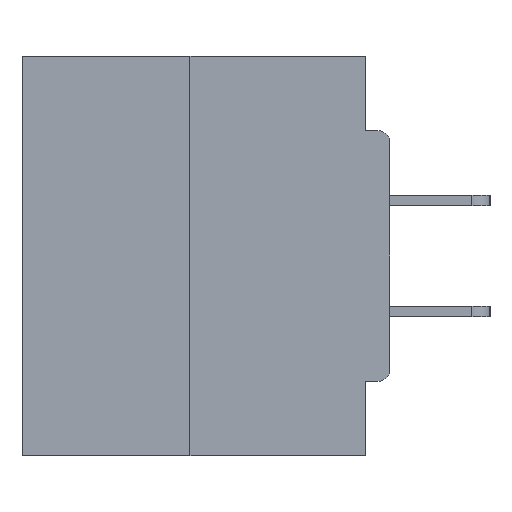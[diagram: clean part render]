
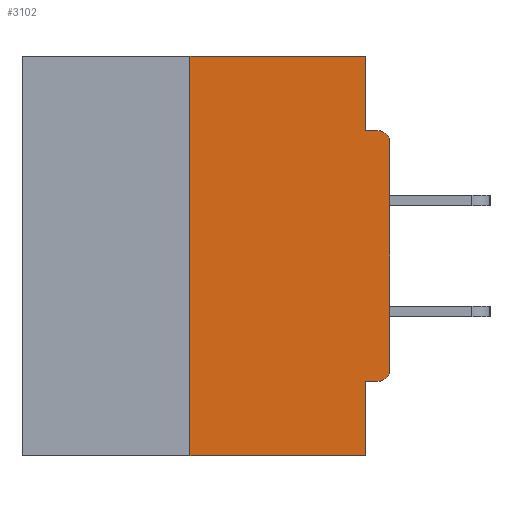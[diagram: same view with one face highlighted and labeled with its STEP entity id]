
A CAD part, left-side view. The second image highlights one B-rep face of the part: STEP entity #3102.
In plain terms, the highlighted planar face has unit normal (-1, 0, 0).
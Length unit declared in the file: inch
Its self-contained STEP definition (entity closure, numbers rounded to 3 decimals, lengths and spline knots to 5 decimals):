
#105 = EDGE_LOOP ( 'NONE', ( #26578, #10068, #1638, #13480, #15799, #30002, #30444, #18837, #18496, #21666 ) ) ;
#568 = VECTOR ( 'NONE', #23103, 39.37008 ) ;
#689 = VERTEX_POINT ( 'NONE', #4109 ) ;
#724 = CARTESIAN_POINT ( 'NONE',  ( 0., 0.25, 0. ) ) ;
#1246 = EDGE_CURVE ( 'NONE', #19488, #25103, #13029, .T. ) ;
#1638 = ORIENTED_EDGE ( 'NONE', *, *, #1246, .T. ) ;
#1678 = CARTESIAN_POINT ( 'NONE',  ( 0., 0., -0.0935 ) ) ;
#2114 = CARTESIAN_POINT ( 'NONE',  ( 0., 0., 0. ) ) ;
#2347 = EDGE_CURVE ( 'NONE', #27531, #13583, #29552, .T. ) ;
#2487 = PLANE ( 'NONE',  #12748 ) ;
#2665 = DIRECTION ( 'NONE',  ( 1., 0., 0. ) ) ;
#3102 = ADVANCED_FACE ( 'NONE', ( #26243 ), #2487, .F. ) ;
#3165 = LINE ( 'NONE', #3693, #26466 ) ;
#3693 = CARTESIAN_POINT ( 'NONE',  ( 0., 0.031, 0. ) ) ;
#4109 = CARTESIAN_POINT ( 'NONE',  ( 0., 0.031, -0.0935 ) ) ;
#5066 = VERTEX_POINT ( 'NONE', #24060 ) ;
#5721 = DIRECTION ( 'NONE',  ( 0., -1., 0. ) ) ;
#5900 = LINE ( 'NONE', #11263, #16922 ) ;
#7303 = VECTOR ( 'NONE', #26386, 39.37008 ) ;
#7584 = EDGE_CURVE ( 'NONE', #689, #13583, #29441, .T. ) ;
#8002 = CARTESIAN_POINT ( 'NONE',  ( 0., 0.25, 0. ) ) ;
#8520 = EDGE_CURVE ( 'NONE', #19488, #20457, #28797, .T. ) ;
#8744 = CARTESIAN_POINT ( 'NONE',  ( 0., 0.031, -0.5 ) ) ;
#9273 = DIRECTION ( 'NONE',  ( 0., -1., 0. ) ) ;
#10068 = ORIENTED_EDGE ( 'NONE', *, *, #8520, .F. ) ;
#10491 = DIRECTION ( 'NONE',  ( -1., 0., 0. ) ) ;
#10493 = LINE ( 'NONE', #29186, #11736 ) ;
#11263 = CARTESIAN_POINT ( 'NONE',  ( 0., 0., -0.4065 ) ) ;
#11736 = VECTOR ( 'NONE', #21068, 39.37008 ) ;
#12113 = EDGE_CURVE ( 'NONE', #5066, #27531, #31227, .T. ) ;
#12748 = AXIS2_PLACEMENT_3D ( 'NONE', #28998, #2665, #21218 ) ;
#13029 = LINE ( 'NONE', #28972, #7303 ) ;
#13480 = ORIENTED_EDGE ( 'NONE', *, *, #18643, .F. ) ;
#13491 = CARTESIAN_POINT ( 'NONE',  ( 0., 0.031, -0.4065 ) ) ;
#13583 = VERTEX_POINT ( 'NONE', #26295 ) ;
#13839 = DIRECTION ( 'NONE',  ( 0., 0., -1. ) ) ;
#14180 = EDGE_CURVE ( 'NONE', #20457, #19867, #14981, .T. ) ;
#14526 = CARTESIAN_POINT ( 'NONE',  ( 0., 0.25, -0.5 ) ) ;
#14981 = LINE ( 'NONE', #30594, #15651 ) ;
#15189 = AXIS2_PLACEMENT_3D ( 'NONE', #22161, #27546, #13839 ) ;
#15651 = VECTOR ( 'NONE', #9273, 39.37008 ) ;
#15670 = VERTEX_POINT ( 'NONE', #13491 ) ;
#15726 = VERTEX_POINT ( 'NONE', #21639 ) ;
#15799 = ORIENTED_EDGE ( 'NONE', *, *, #23806, .F. ) ;
#16472 = CARTESIAN_POINT ( 'NONE',  ( 0., 0., -0.1085 ) ) ;
#16922 = VECTOR ( 'NONE', #21325, 39.37008 ) ;
#18496 = ORIENTED_EDGE ( 'NONE', *, *, #7584, .F. ) ;
#18643 = EDGE_CURVE ( 'NONE', #15670, #25103, #10493, .T. ) ;
#18837 = ORIENTED_EDGE ( 'NONE', *, *, #2347, .T. ) ;
#19265 = DIRECTION ( 'NONE',  ( 0., 0., 1. ) ) ;
#19488 = VERTEX_POINT ( 'NONE', #14526 ) ;
#19867 = VERTEX_POINT ( 'NONE', #29363 ) ;
#20457 = VERTEX_POINT ( 'NONE', #724 ) ;
#20562 = DIRECTION ( 'NONE',  ( 0., 0., -1. ) ) ;
#21068 = DIRECTION ( 'NONE',  ( 0., 0., -1. ) ) ;
#21218 = DIRECTION ( 'NONE',  ( 0., 0., -1. ) ) ;
#21325 = DIRECTION ( 'NONE',  ( 0., 1., 0. ) ) ;
#21639 = CARTESIAN_POINT ( 'NONE',  ( 0., 0.015, -0.4065 ) ) ;
#21666 = ORIENTED_EDGE ( 'NONE', *, *, #33200, .F. ) ;
#22161 = CARTESIAN_POINT ( 'NONE',  ( 0., 0.015, -0.1085 ) ) ;
#23103 = DIRECTION ( 'NONE',  ( 0., 0., 1. ) ) ;
#23223 = VECTOR ( 'NONE', #19265, 39.37008 ) ;
#23806 = EDGE_CURVE ( 'NONE', #15726, #15670, #5900, .T. ) ;
#24060 = CARTESIAN_POINT ( 'NONE',  ( 0., 0., -0.3915 ) ) ;
#24362 = VECTOR ( 'NONE', #5721, 39.37008 ) ;
#24860 = DIRECTION ( 'NONE',  ( 0., 0., -1. ) ) ;
#24895 = EDGE_CURVE ( 'NONE', #15726, #5066, #31900, .T. ) ;
#25103 = VERTEX_POINT ( 'NONE', #8744 ) ;
#26243 = FACE_OUTER_BOUND ( 'NONE', #105, .T. ) ;
#26295 = CARTESIAN_POINT ( 'NONE',  ( 0., 0.015, -0.0935 ) ) ;
#26386 = DIRECTION ( 'NONE',  ( 0., -1., 0. ) ) ;
#26466 = VECTOR ( 'NONE', #24860, 39.37008 ) ;
#26578 = ORIENTED_EDGE ( 'NONE', *, *, #14180, .F. ) ;
#27531 = VERTEX_POINT ( 'NONE', #16472 ) ;
#27546 = DIRECTION ( 'NONE',  ( -1., 0., 0. ) ) ;
#28367 = CARTESIAN_POINT ( 'NONE',  ( 0., 0.015, -0.3915 ) ) ;
#28797 = LINE ( 'NONE', #8002, #23223 ) ;
#28972 = CARTESIAN_POINT ( 'NONE',  ( 0., 0.46, -0.5 ) ) ;
#28998 = CARTESIAN_POINT ( 'NONE',  ( 0., 0.46, 0. ) ) ;
#29186 = CARTESIAN_POINT ( 'NONE',  ( 0., 0.031, -0.5 ) ) ;
#29363 = CARTESIAN_POINT ( 'NONE',  ( 0., 0.031, 0. ) ) ;
#29441 = LINE ( 'NONE', #1678, #24362 ) ;
#29552 = CIRCLE ( 'NONE', #15189, 0.015 ) ;
#30002 = ORIENTED_EDGE ( 'NONE', *, *, #24895, .T. ) ;
#30444 = ORIENTED_EDGE ( 'NONE', *, *, #12113, .T. ) ;
#30594 = CARTESIAN_POINT ( 'NONE',  ( 0., 0.46, 0. ) ) ;
#31227 = LINE ( 'NONE', #2114, #568 ) ;
#31900 = CIRCLE ( 'NONE', #34138, 0.015 ) ;
#33200 = EDGE_CURVE ( 'NONE', #19867, #689, #3165, .T. ) ;
#34138 = AXIS2_PLACEMENT_3D ( 'NONE', #28367, #10491, #20562 ) ;
